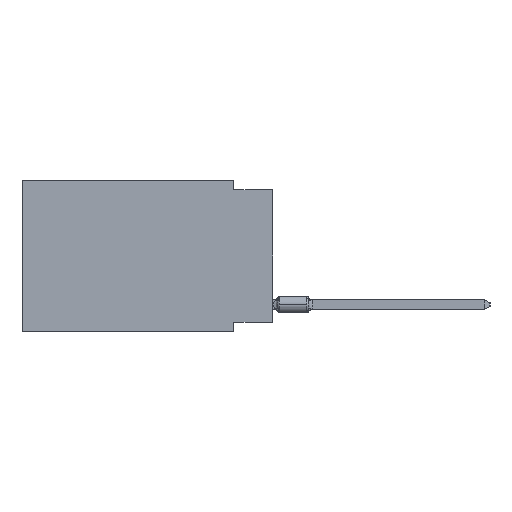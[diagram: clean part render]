
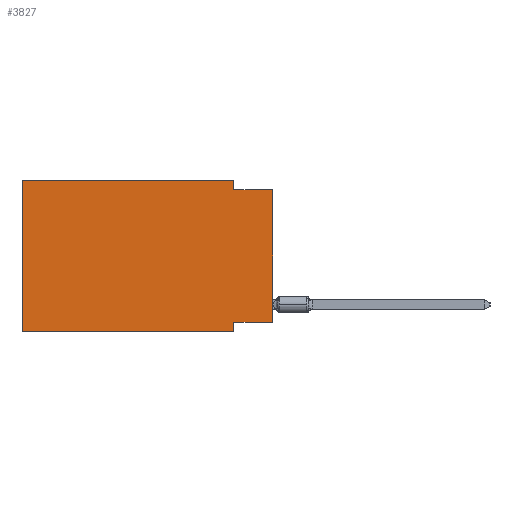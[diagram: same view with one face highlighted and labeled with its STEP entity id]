
A CAD part, left-side view. The second image highlights one B-rep face of the part: STEP entity #3827.
In plain terms, the highlighted planar face has unit normal (-1, 0, 0).
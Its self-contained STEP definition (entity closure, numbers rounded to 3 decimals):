
#280 = CARTESIAN_POINT ( 'NONE',  ( 0., 16.383, -9.906 ) ) ;
#1220 = VECTOR ( 'NONE', #13015, 1000. ) ;
#3693 = LINE ( 'NONE', #21303, #23029 ) ;
#3827 = ADVANCED_FACE ( 'NONE', ( #26914 ), #18575, .F. ) ;
#4476 = LINE ( 'NONE', #9803, #1220 ) ;
#4772 = VECTOR ( 'NONE', #22185, 1000. ) ;
#6139 = DIRECTION ( 'NONE',  ( 0., 0., 1. ) ) ;
#6255 = EDGE_CURVE ( 'NONE', #28270, #19605, #7796, .T. ) ;
#6903 = DIRECTION ( 'NONE',  ( 0., 0., 1. ) ) ;
#6957 = CARTESIAN_POINT ( 'NONE',  ( 0., 2.54, -0.635 ) ) ;
#6996 = VERTEX_POINT ( 'NONE', #6957 ) ;
#7337 = CARTESIAN_POINT ( 'NONE',  ( 0., 16.383, 0. ) ) ;
#7498 = ORIENTED_EDGE ( 'NONE', *, *, #16160, .T. ) ;
#7796 = LINE ( 'NONE', #13887, #4772 ) ;
#7818 = ORIENTED_EDGE ( 'NONE', *, *, #23981, .F. ) ;
#7890 = ORIENTED_EDGE ( 'NONE', *, *, #21675, .F. ) ;
#8740 = ORIENTED_EDGE ( 'NONE', *, *, #20101, .F. ) ;
#9133 = CARTESIAN_POINT ( 'NONE',  ( 0., 0., -9.271 ) ) ;
#9557 = CARTESIAN_POINT ( 'NONE',  ( 0., 2.54, -9.906 ) ) ;
#9613 = DIRECTION ( 'NONE',  ( 0., -1., 0. ) ) ;
#9803 = CARTESIAN_POINT ( 'NONE',  ( 0., 2.54, 0. ) ) ;
#9922 = CARTESIAN_POINT ( 'NONE',  ( 0., 16.383, -9.906 ) ) ;
#10044 = DIRECTION ( 'NONE',  ( 0., 0., -1. ) ) ;
#11646 = LINE ( 'NONE', #34568, #16511 ) ;
#11974 = EDGE_CURVE ( 'NONE', #28971, #26445, #27707, .T. ) ;
#12111 = LINE ( 'NONE', #35213, #12674 ) ;
#12674 = VECTOR ( 'NONE', #18357, 1000. ) ;
#13015 = DIRECTION ( 'NONE',  ( 0., 0., -1. ) ) ;
#13545 = CARTESIAN_POINT ( 'NONE',  ( 0., 2.54, -9.271 ) ) ;
#13887 = CARTESIAN_POINT ( 'NONE',  ( 0., 0., -9.271 ) ) ;
#14897 = ORIENTED_EDGE ( 'NONE', *, *, #15742, .F. ) ;
#15191 = EDGE_LOOP ( 'NONE', ( #7498, #8740, #14897, #7818, #7890, #27659, #31614, #33039 ) ) ;
#15295 = VECTOR ( 'NONE', #15607, 1000. ) ;
#15607 = DIRECTION ( 'NONE',  ( 0., -1., 0. ) ) ;
#15742 = EDGE_CURVE ( 'NONE', #17357, #6996, #4476, .T. ) ;
#16160 = EDGE_CURVE ( 'NONE', #28270, #32853, #3693, .T. ) ;
#16511 = VECTOR ( 'NONE', #6139, 1000. ) ;
#17357 = VERTEX_POINT ( 'NONE', #23592 ) ;
#18240 = EDGE_CURVE ( 'NONE', #19605, #26445, #12111, .T. ) ;
#18357 = DIRECTION ( 'NONE',  ( 0., 0., -1. ) ) ;
#18575 = PLANE ( 'NONE',  #20365 ) ;
#19013 = CARTESIAN_POINT ( 'NONE',  ( 0., 0., -0.635 ) ) ;
#19605 = VERTEX_POINT ( 'NONE', #13545 ) ;
#20101 = EDGE_CURVE ( 'NONE', #6996, #32853, #25210, .T. ) ;
#20365 = AXIS2_PLACEMENT_3D ( 'NONE', #29939, #35992, #10044 ) ;
#21303 = CARTESIAN_POINT ( 'NONE',  ( 0., 0., 0. ) ) ;
#21355 = LINE ( 'NONE', #7337, #29650 ) ;
#21675 = EDGE_CURVE ( 'NONE', #28971, #36456, #11646, .T. ) ;
#22185 = DIRECTION ( 'NONE',  ( 0., 1., 0. ) ) ;
#23029 = VECTOR ( 'NONE', #6903, 1000. ) ;
#23070 = VECTOR ( 'NONE', #25607, 1000. ) ;
#23592 = CARTESIAN_POINT ( 'NONE',  ( 0., 2.54, 0. ) ) ;
#23981 = EDGE_CURVE ( 'NONE', #36456, #17357, #21355, .T. ) ;
#25210 = LINE ( 'NONE', #28818, #23070 ) ;
#25607 = DIRECTION ( 'NONE',  ( 0., -1., 0. ) ) ;
#26445 = VERTEX_POINT ( 'NONE', #9557 ) ;
#26914 = FACE_OUTER_BOUND ( 'NONE', #15191, .T. ) ;
#27659 = ORIENTED_EDGE ( 'NONE', *, *, #11974, .T. ) ;
#27707 = LINE ( 'NONE', #9922, #15295 ) ;
#28082 = CARTESIAN_POINT ( 'NONE',  ( 0., 16.383, 0. ) ) ;
#28270 = VERTEX_POINT ( 'NONE', #9133 ) ;
#28818 = CARTESIAN_POINT ( 'NONE',  ( 0., 0., -0.635 ) ) ;
#28971 = VERTEX_POINT ( 'NONE', #280 ) ;
#29650 = VECTOR ( 'NONE', #9613, 1000. ) ;
#29939 = CARTESIAN_POINT ( 'NONE',  ( 0., 16.383, 0. ) ) ;
#31614 = ORIENTED_EDGE ( 'NONE', *, *, #18240, .F. ) ;
#32853 = VERTEX_POINT ( 'NONE', #19013 ) ;
#33039 = ORIENTED_EDGE ( 'NONE', *, *, #6255, .F. ) ;
#34568 = CARTESIAN_POINT ( 'NONE',  ( 0., 16.383, 0. ) ) ;
#35213 = CARTESIAN_POINT ( 'NONE',  ( 0., 2.54, -9.906 ) ) ;
#35992 = DIRECTION ( 'NONE',  ( 1., 0., 0. ) ) ;
#36456 = VERTEX_POINT ( 'NONE', #28082 ) ;
